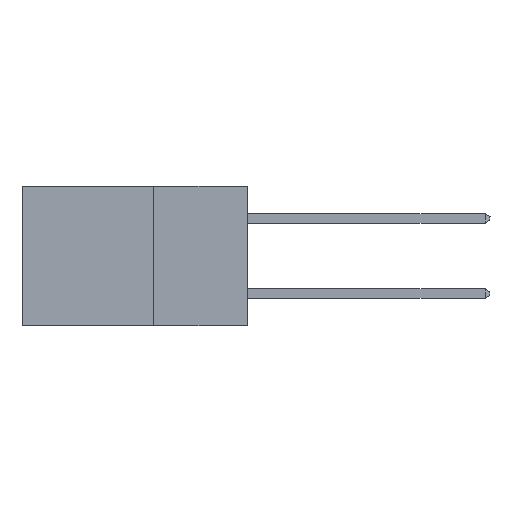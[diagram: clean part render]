
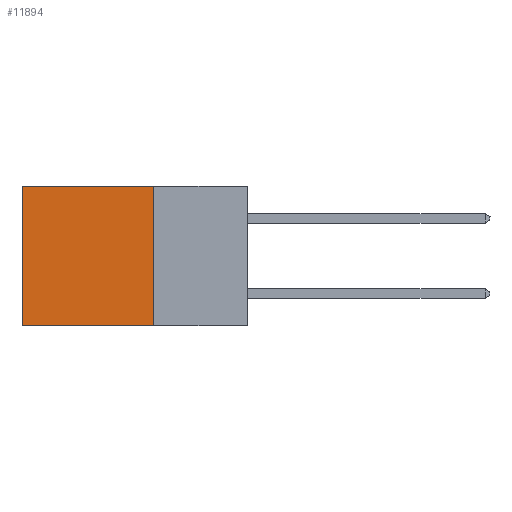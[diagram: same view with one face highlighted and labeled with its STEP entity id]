
A CAD part, left-side view. The second image highlights one B-rep face of the part: STEP entity #11894.
In plain terms, the highlighted planar face has unit normal (-1, 0, 0).
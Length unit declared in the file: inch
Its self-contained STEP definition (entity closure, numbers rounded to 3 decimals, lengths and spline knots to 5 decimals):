
#865 = CARTESIAN_POINT ( 'NONE',  ( 0.298, 0.25, -0.37 ) ) ;
#1229 = VECTOR ( 'NONE', #9037, 39.37008 ) ;
#1803 = ORIENTED_EDGE ( 'NONE', *, *, #19106, .T. ) ;
#2223 = CARTESIAN_POINT ( 'NONE',  ( 0.298, 0.25, -0.37 ) ) ;
#2495 = DIRECTION ( 'NONE',  ( 0., 1., 0. ) ) ;
#2711 = ORIENTED_EDGE ( 'NONE', *, *, #3317, .F. ) ;
#2765 = CARTESIAN_POINT ( 'NONE',  ( 0.298, 0.25, 0. ) ) ;
#3317 = EDGE_CURVE ( 'NONE', #17638, #3829, #19697, .T. ) ;
#3744 = CARTESIAN_POINT ( 'NONE',  ( 0.298, 0.6, 0. ) ) ;
#3829 = VERTEX_POINT ( 'NONE', #4260 ) ;
#4015 = EDGE_CURVE ( 'NONE', #4825, #15210, #9702, .T. ) ;
#4260 = CARTESIAN_POINT ( 'NONE',  ( 0.298, 0.6, -0.37 ) ) ;
#4825 = VERTEX_POINT ( 'NONE', #2765 ) ;
#5100 = FACE_OUTER_BOUND ( 'NONE', #5167, .T. ) ;
#5167 = EDGE_LOOP ( 'NONE', ( #1803, #2711, #15481, #16447 ) ) ;
#6329 = LINE ( 'NONE', #17771, #9534 ) ;
#6491 = PLANE ( 'NONE',  #7227 ) ;
#7227 = AXIS2_PLACEMENT_3D ( 'NONE', #17420, #18989, #9655 ) ;
#9037 = DIRECTION ( 'NONE',  ( 0., 1., 0. ) ) ;
#9534 = VECTOR ( 'NONE', #9987, 39.37008 ) ;
#9655 = DIRECTION ( 'NONE',  ( 0., 0., -1. ) ) ;
#9702 = LINE ( 'NONE', #12216, #1229 ) ;
#9987 = DIRECTION ( 'NONE',  ( 0., 0., -1. ) ) ;
#11630 = VECTOR ( 'NONE', #20078, 39.37008 ) ;
#11894 = ADVANCED_FACE ( 'NONE', ( #5100 ), #6491, .F. ) ;
#12060 = EDGE_CURVE ( 'NONE', #4825, #17638, #6329, .T. ) ;
#12216 = CARTESIAN_POINT ( 'NONE',  ( 0.298, 0.25, 0. ) ) ;
#15117 = VECTOR ( 'NONE', #2495, 39.37008 ) ;
#15210 = VERTEX_POINT ( 'NONE', #3744 ) ;
#15481 = ORIENTED_EDGE ( 'NONE', *, *, #12060, .F. ) ;
#15760 = LINE ( 'NONE', #16985, #11630 ) ;
#16447 = ORIENTED_EDGE ( 'NONE', *, *, #4015, .T. ) ;
#16985 = CARTESIAN_POINT ( 'NONE',  ( 0.298, 0.6, 0. ) ) ;
#17420 = CARTESIAN_POINT ( 'NONE',  ( 0.298, 0.25, 0. ) ) ;
#17638 = VERTEX_POINT ( 'NONE', #865 ) ;
#17771 = CARTESIAN_POINT ( 'NONE',  ( 0.298, 0.25, 0. ) ) ;
#18989 = DIRECTION ( 'NONE',  ( 1., 0., 0. ) ) ;
#19106 = EDGE_CURVE ( 'NONE', #15210, #3829, #15760, .T. ) ;
#19697 = LINE ( 'NONE', #2223, #15117 ) ;
#20078 = DIRECTION ( 'NONE',  ( 0., 0., -1. ) ) ;
